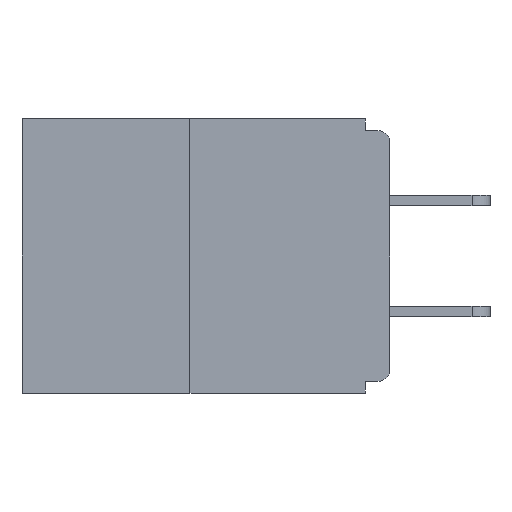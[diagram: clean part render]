
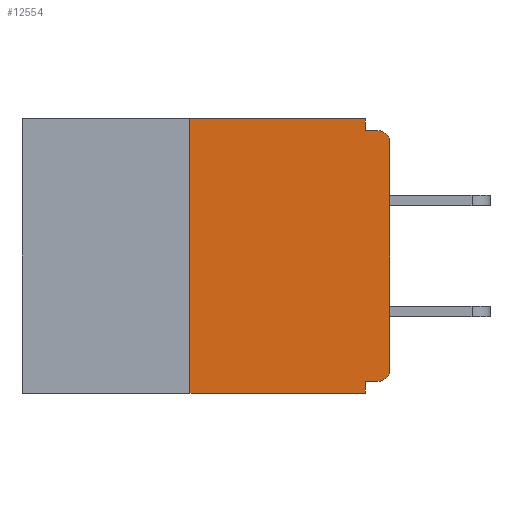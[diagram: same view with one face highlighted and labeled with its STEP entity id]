
A CAD part, left-side view. The second image highlights one B-rep face of the part: STEP entity #12554.
In plain terms, the highlighted planar face has unit normal (-1, 0, 0).
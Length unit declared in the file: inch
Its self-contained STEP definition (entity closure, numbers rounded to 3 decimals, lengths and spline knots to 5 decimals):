
#654 = ORIENTED_EDGE ( 'NONE', *, *, #22224, .F. ) ;
#692 = CARTESIAN_POINT ( 'NONE',  ( 0., 0.015, -0.313 ) ) ;
#1269 = ORIENTED_EDGE ( 'NONE', *, *, #4645, .T. ) ;
#1287 = VERTEX_POINT ( 'NONE', #21452 ) ;
#1785 = LINE ( 'NONE', #19904, #13740 ) ;
#2038 = CARTESIAN_POINT ( 'NONE',  ( 0., 0.46, 0. ) ) ;
#2361 = LINE ( 'NONE', #2473, #6947 ) ;
#2442 = VECTOR ( 'NONE', #27905, 39.37008 ) ;
#2473 = CARTESIAN_POINT ( 'NONE',  ( 0., 0.25, 0. ) ) ;
#2866 = CARTESIAN_POINT ( 'NONE',  ( 0., 0., 0. ) ) ;
#3158 = ORIENTED_EDGE ( 'NONE', *, *, #11335, .T. ) ;
#3593 = DIRECTION ( 'NONE',  ( 0., 0., -1. ) ) ;
#3942 = DIRECTION ( 'NONE',  ( 0., -1., 0. ) ) ;
#4324 = DIRECTION ( 'NONE',  ( 0., -1., 0. ) ) ;
#4645 = EDGE_CURVE ( 'NONE', #1287, #5467, #1785, .T. ) ;
#4926 = VERTEX_POINT ( 'NONE', #25551 ) ;
#5007 = CARTESIAN_POINT ( 'NONE',  ( 0., 0.031, -0.343 ) ) ;
#5166 = CARTESIAN_POINT ( 'NONE',  ( 0., 0., -0.03 ) ) ;
#5467 = VERTEX_POINT ( 'NONE', #28615 ) ;
#5584 = CARTESIAN_POINT ( 'NONE',  ( 0., 0.015, -0.03 ) ) ;
#6225 = CARTESIAN_POINT ( 'NONE',  ( 0., 0.46, 0. ) ) ;
#6941 = DIRECTION ( 'NONE',  ( 0., 0., -1. ) ) ;
#6947 = VECTOR ( 'NONE', #18260, 39.37008 ) ;
#7277 = DIRECTION ( 'NONE',  ( 0., 0., -1. ) ) ;
#7608 = EDGE_CURVE ( 'NONE', #4926, #27851, #15465, .T. ) ;
#7869 = CIRCLE ( 'NONE', #16791, 0.015 ) ;
#8352 = FACE_OUTER_BOUND ( 'NONE', #24896, .T. ) ;
#10550 = LINE ( 'NONE', #2866, #2442 ) ;
#10562 = EDGE_CURVE ( 'NONE', #22213, #18436, #7869, .T. ) ;
#10736 = AXIS2_PLACEMENT_3D ( 'NONE', #2038, #17924, #26583 ) ;
#10911 = CARTESIAN_POINT ( 'NONE',  ( 0., 0., -0.328 ) ) ;
#11151 = ORIENTED_EDGE ( 'NONE', *, *, #10562, .T. ) ;
#11335 = EDGE_CURVE ( 'NONE', #13763, #27587, #24110, .T. ) ;
#11591 = VECTOR ( 'NONE', #6941, 39.37008 ) ;
#12554 = ADVANCED_FACE ( 'NONE', ( #8352 ), #15531, .F. ) ;
#12809 = ORIENTED_EDGE ( 'NONE', *, *, #7608, .F. ) ;
#12810 = VERTEX_POINT ( 'NONE', #16820 ) ;
#13634 = CARTESIAN_POINT ( 'NONE',  ( 0., 0.031, -0.015 ) ) ;
#13740 = VECTOR ( 'NONE', #17612, 39.37008 ) ;
#13763 = VERTEX_POINT ( 'NONE', #5166 ) ;
#14560 = DIRECTION ( 'NONE',  ( -1., 0., 0. ) ) ;
#14733 = CARTESIAN_POINT ( 'NONE',  ( 0., 0., -0.313 ) ) ;
#14878 = ORIENTED_EDGE ( 'NONE', *, *, #21602, .F. ) ;
#15465 = LINE ( 'NONE', #22660, #11591 ) ;
#15531 = PLANE ( 'NONE',  #10736 ) ;
#16791 = AXIS2_PLACEMENT_3D ( 'NONE', #692, #14560, #18962 ) ;
#16820 = CARTESIAN_POINT ( 'NONE',  ( 0., 0.031, -0.328 ) ) ;
#17183 = CARTESIAN_POINT ( 'NONE',  ( 0., 0.015, -0.328 ) ) ;
#17339 = CARTESIAN_POINT ( 'NONE',  ( 0., 0.015, -0.015 ) ) ;
#17360 = VECTOR ( 'NONE', #7277, 39.37008 ) ;
#17392 = ORIENTED_EDGE ( 'NONE', *, *, #28344, .F. ) ;
#17612 = DIRECTION ( 'NONE',  ( 0., -1., 0. ) ) ;
#17849 = VERTEX_POINT ( 'NONE', #27705 ) ;
#17924 = DIRECTION ( 'NONE',  ( 1., 0., 0. ) ) ;
#17954 = LINE ( 'NONE', #10911, #25040 ) ;
#18253 = LINE ( 'NONE', #6225, #22874 ) ;
#18260 = DIRECTION ( 'NONE',  ( 0., 0., 1. ) ) ;
#18436 = VERTEX_POINT ( 'NONE', #14733 ) ;
#18694 = AXIS2_PLACEMENT_3D ( 'NONE', #5584, #28409, #3593 ) ;
#18962 = DIRECTION ( 'NONE',  ( 0., 0., -1. ) ) ;
#19323 = ORIENTED_EDGE ( 'NONE', *, *, #20057, .F. ) ;
#19677 = LINE ( 'NONE', #29142, #24272 ) ;
#19904 = CARTESIAN_POINT ( 'NONE',  ( 0., 0.46, -0.343 ) ) ;
#20038 = DIRECTION ( 'NONE',  ( 0., 1., 0. ) ) ;
#20057 = EDGE_CURVE ( 'NONE', #12810, #5467, #23399, .T. ) ;
#21452 = CARTESIAN_POINT ( 'NONE',  ( 0., 0.25, -0.343 ) ) ;
#21602 = EDGE_CURVE ( 'NONE', #22213, #12810, #17954, .T. ) ;
#22213 = VERTEX_POINT ( 'NONE', #17183 ) ;
#22224 = EDGE_CURVE ( 'NONE', #17849, #4926, #18253, .T. ) ;
#22660 = CARTESIAN_POINT ( 'NONE',  ( 0., 0.031, 0. ) ) ;
#22759 = EDGE_CURVE ( 'NONE', #27851, #27587, #19677, .T. ) ;
#22874 = VECTOR ( 'NONE', #3942, 39.37008 ) ;
#23399 = LINE ( 'NONE', #5007, #17360 ) ;
#24110 = CIRCLE ( 'NONE', #18694, 0.015 ) ;
#24272 = VECTOR ( 'NONE', #4324, 39.37008 ) ;
#24477 = ORIENTED_EDGE ( 'NONE', *, *, #26058, .T. ) ;
#24896 = EDGE_LOOP ( 'NONE', ( #654, #17392, #1269, #19323, #14878, #11151, #24477, #3158, #25644, #12809 ) ) ;
#25040 = VECTOR ( 'NONE', #20038, 39.37008 ) ;
#25551 = CARTESIAN_POINT ( 'NONE',  ( 0., 0.031, 0. ) ) ;
#25644 = ORIENTED_EDGE ( 'NONE', *, *, #22759, .F. ) ;
#26058 = EDGE_CURVE ( 'NONE', #18436, #13763, #10550, .T. ) ;
#26583 = DIRECTION ( 'NONE',  ( 0., 0., -1. ) ) ;
#27587 = VERTEX_POINT ( 'NONE', #17339 ) ;
#27705 = CARTESIAN_POINT ( 'NONE',  ( 0., 0.25, 0. ) ) ;
#27851 = VERTEX_POINT ( 'NONE', #13634 ) ;
#27905 = DIRECTION ( 'NONE',  ( 0., 0., 1. ) ) ;
#28344 = EDGE_CURVE ( 'NONE', #1287, #17849, #2361, .T. ) ;
#28409 = DIRECTION ( 'NONE',  ( -1., 0., 0. ) ) ;
#28615 = CARTESIAN_POINT ( 'NONE',  ( 0., 0.031, -0.343 ) ) ;
#29142 = CARTESIAN_POINT ( 'NONE',  ( 0., 0., -0.015 ) ) ;
